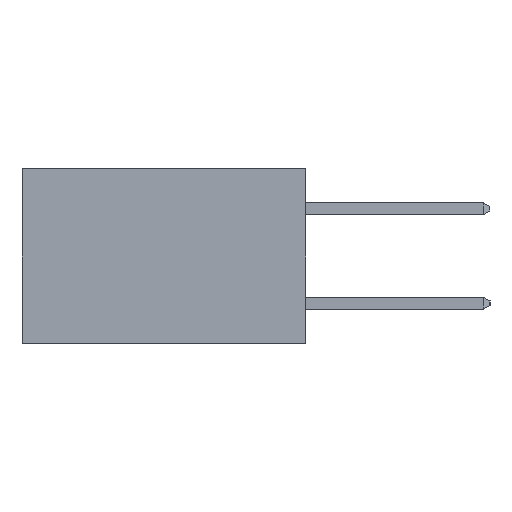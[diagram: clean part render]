
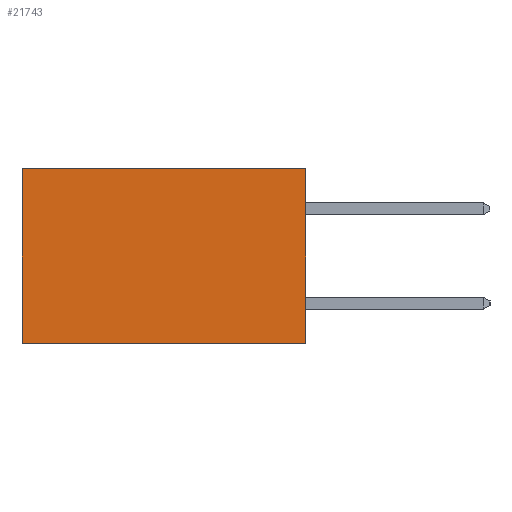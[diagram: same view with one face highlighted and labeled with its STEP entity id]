
A CAD part, left-side view. The second image highlights one B-rep face of the part: STEP entity #21743.
In plain terms, the highlighted planar face has unit normal (-1, 0, 0).
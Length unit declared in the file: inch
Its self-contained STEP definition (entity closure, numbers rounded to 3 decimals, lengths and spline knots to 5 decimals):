
#3 = EDGE_CURVE ( 'NONE', #25385, #3953, #17387, .T. ) ;
#1100 = CARTESIAN_POINT ( 'NONE',  ( 0.2615, 0., -0.37 ) ) ;
#1449 = VERTEX_POINT ( 'NONE', #9861 ) ;
#2127 = CARTESIAN_POINT ( 'NONE',  ( 0.2615, 0., -0.37 ) ) ;
#2987 = AXIS2_PLACEMENT_3D ( 'NONE', #1100, #15184, #3160 ) ;
#3160 = DIRECTION ( 'NONE',  ( 0., 0., -1. ) ) ;
#3510 = LINE ( 'NONE', #2127, #8913 ) ;
#3721 = ORIENTED_EDGE ( 'NONE', *, *, #25660, .F. ) ;
#3953 = VERTEX_POINT ( 'NONE', #10512 ) ;
#6755 = VECTOR ( 'NONE', #18475, 39.37008 ) ;
#8913 = VECTOR ( 'NONE', #14195, 39.37008 ) ;
#8920 = ORIENTED_EDGE ( 'NONE', *, *, #17709, .T. ) ;
#9039 = VECTOR ( 'NONE', #19793, 39.37008 ) ;
#9861 = CARTESIAN_POINT ( 'NONE',  ( 0.2615, 0.6, 0. ) ) ;
#10512 = CARTESIAN_POINT ( 'NONE',  ( 0.2615, 0.6, -0.37 ) ) ;
#10610 = CARTESIAN_POINT ( 'NONE',  ( 0.2615, 0.6, -0.37 ) ) ;
#11898 = CARTESIAN_POINT ( 'NONE',  ( 0.2615, 0., 0. ) ) ;
#12093 = VECTOR ( 'NONE', #21012, 39.37008 ) ;
#14195 = DIRECTION ( 'NONE',  ( 0., 0., -1. ) ) ;
#15071 = CARTESIAN_POINT ( 'NONE',  ( 0.2615, 0., 0. ) ) ;
#15184 = DIRECTION ( 'NONE',  ( 1., 0., 0. ) ) ;
#16453 = VERTEX_POINT ( 'NONE', #15071 ) ;
#16779 = CARTESIAN_POINT ( 'NONE',  ( 0.2615, 0., -0.37 ) ) ;
#17387 = LINE ( 'NONE', #16779, #12093 ) ;
#17709 = EDGE_CURVE ( 'NONE', #1449, #3953, #21995, .T. ) ;
#18077 = ORIENTED_EDGE ( 'NONE', *, *, #3, .F. ) ;
#18475 = DIRECTION ( 'NONE',  ( 0., 0., -1. ) ) ;
#18958 = ORIENTED_EDGE ( 'NONE', *, *, #22839, .T. ) ;
#19603 = LINE ( 'NONE', #11898, #9039 ) ;
#19793 = DIRECTION ( 'NONE',  ( 0., 1., 0. ) ) ;
#20900 = PLANE ( 'NONE',  #2987 ) ;
#21012 = DIRECTION ( 'NONE',  ( 0., 1., 0. ) ) ;
#21649 = CARTESIAN_POINT ( 'NONE',  ( 0.2615, 0., -0.37 ) ) ;
#21743 = ADVANCED_FACE ( 'NONE', ( #25701 ), #20900, .F. ) ;
#21995 = LINE ( 'NONE', #10610, #6755 ) ;
#22839 = EDGE_CURVE ( 'NONE', #16453, #1449, #19603, .T. ) ;
#24594 = EDGE_LOOP ( 'NONE', ( #8920, #18077, #3721, #18958 ) ) ;
#25385 = VERTEX_POINT ( 'NONE', #21649 ) ;
#25660 = EDGE_CURVE ( 'NONE', #16453, #25385, #3510, .T. ) ;
#25701 = FACE_OUTER_BOUND ( 'NONE', #24594, .T. ) ;
